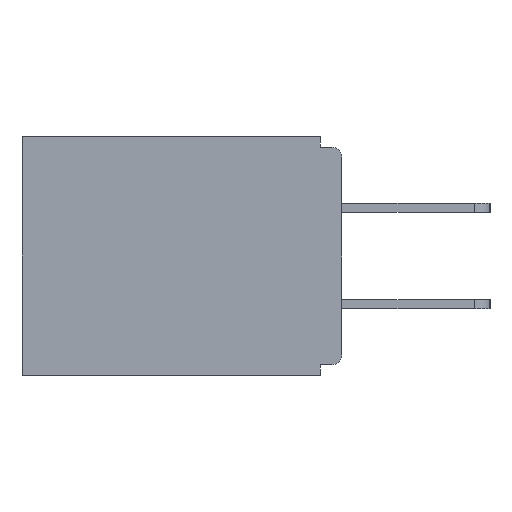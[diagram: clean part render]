
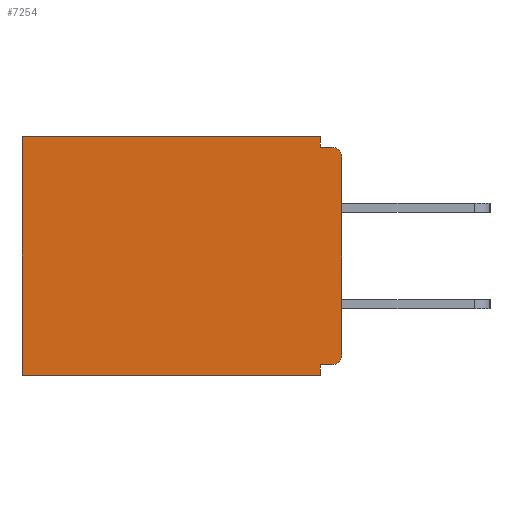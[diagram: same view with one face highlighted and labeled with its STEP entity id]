
A CAD part, left-side view. The second image highlights one B-rep face of the part: STEP entity #7254.
In plain terms, the highlighted planar face has unit normal (-1, 0, 0).
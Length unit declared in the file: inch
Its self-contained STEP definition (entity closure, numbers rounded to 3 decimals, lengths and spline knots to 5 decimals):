
#110 = VECTOR ( 'NONE', #3729, 39.37008 ) ;
#126 = VERTEX_POINT ( 'NONE', #10903 ) ;
#396 = DIRECTION ( 'NONE',  ( 1., 0., 0. ) ) ;
#443 = ORIENTED_EDGE ( 'NONE', *, *, #1362, .F. ) ;
#806 = CIRCLE ( 'NONE', #9338, 0.015 ) ;
#890 = VECTOR ( 'NONE', #6838, 39.37008 ) ;
#956 = VERTEX_POINT ( 'NONE', #1411 ) ;
#1042 = DIRECTION ( 'NONE',  ( 0., 1., 0. ) ) ;
#1362 = EDGE_CURVE ( 'NONE', #8880, #956, #7455, .T. ) ;
#1411 = CARTESIAN_POINT ( 'NONE',  ( 0.298, 0.015, -0.015 ) ) ;
#1448 = VERTEX_POINT ( 'NONE', #7820 ) ;
#1526 = AXIS2_PLACEMENT_3D ( 'NONE', #4943, #396, #4019 ) ;
#1796 = ORIENTED_EDGE ( 'NONE', *, *, #1849, .F. ) ;
#1849 = EDGE_CURVE ( 'NONE', #6363, #6569, #5545, .T. ) ;
#1912 = LINE ( 'NONE', #2779, #2485 ) ;
#1983 = CARTESIAN_POINT ( 'NONE',  ( 0.298, 0.015, -0.03 ) ) ;
#2081 = CARTESIAN_POINT ( 'NONE',  ( 0.298, 0., -0.343 ) ) ;
#2142 = CARTESIAN_POINT ( 'NONE',  ( 0.298, 0.031, -0.343 ) ) ;
#2427 = CARTESIAN_POINT ( 'NONE',  ( 0.298, 0.031, -0.328 ) ) ;
#2485 = VECTOR ( 'NONE', #1042, 39.37008 ) ;
#2779 = CARTESIAN_POINT ( 'NONE',  ( 0.298, 0., -0.328 ) ) ;
#3305 = ORIENTED_EDGE ( 'NONE', *, *, #5912, .F. ) ;
#3526 = DIRECTION ( 'NONE',  ( -1., 0., 0. ) ) ;
#3548 = EDGE_CURVE ( 'NONE', #1448, #8880, #4647, .T. ) ;
#3716 = AXIS2_PLACEMENT_3D ( 'NONE', #5342, #3526, #5758 ) ;
#3729 = DIRECTION ( 'NONE',  ( 0., 1., 0. ) ) ;
#3808 = CARTESIAN_POINT ( 'NONE',  ( 0.298, 0.015, -0.328 ) ) ;
#3820 = CIRCLE ( 'NONE', #3716, 0.015 ) ;
#3954 = CARTESIAN_POINT ( 'NONE',  ( 0.298, 0., -0.015 ) ) ;
#4019 = DIRECTION ( 'NONE',  ( 0., 0., -1. ) ) ;
#4382 = CARTESIAN_POINT ( 'NONE',  ( 0.298, 0., 0. ) ) ;
#4394 = VECTOR ( 'NONE', #4870, 39.37008 ) ;
#4421 = DIRECTION ( 'NONE',  ( 0., 0., -1. ) ) ;
#4441 = EDGE_CURVE ( 'NONE', #6363, #956, #806, .T. ) ;
#4455 = ORIENTED_EDGE ( 'NONE', *, *, #6949, .T. ) ;
#4647 = LINE ( 'NONE', #2142, #890 ) ;
#4870 = DIRECTION ( 'NONE',  ( 0., 0., -1. ) ) ;
#4943 = CARTESIAN_POINT ( 'NONE',  ( 0.298, 0., 0. ) ) ;
#4975 = VERTEX_POINT ( 'NONE', #8920 ) ;
#5342 = CARTESIAN_POINT ( 'NONE',  ( 0.298, 0.015, -0.313 ) ) ;
#5377 = EDGE_LOOP ( 'NONE', ( #6975, #443, #8109, #9449, #5841, #9059, #7332, #3305, #4455, #1796 ) ) ;
#5424 = CARTESIAN_POINT ( 'NONE',  ( 0.298, 0., -0.313 ) ) ;
#5545 = LINE ( 'NONE', #4382, #7303 ) ;
#5651 = CARTESIAN_POINT ( 'NONE',  ( 0.298, 0.031, -0.343 ) ) ;
#5711 = CARTESIAN_POINT ( 'NONE',  ( 0.298, 0.46, 0. ) ) ;
#5743 = CARTESIAN_POINT ( 'NONE',  ( 0.298, 0., -0.03 ) ) ;
#5758 = DIRECTION ( 'NONE',  ( 0., 0., -1. ) ) ;
#5841 = ORIENTED_EDGE ( 'NONE', *, *, #6872, .T. ) ;
#5912 = EDGE_CURVE ( 'NONE', #7705, #11423, #1912, .T. ) ;
#6060 = DIRECTION ( 'NONE',  ( 0., 1., 0. ) ) ;
#6061 = DIRECTION ( 'NONE',  ( 0., -1., 0. ) ) ;
#6254 = LINE ( 'NONE', #2081, #110 ) ;
#6363 = VERTEX_POINT ( 'NONE', #5743 ) ;
#6384 = EDGE_CURVE ( 'NONE', #126, #4975, #6254, .T. ) ;
#6502 = LINE ( 'NONE', #8766, #7724 ) ;
#6569 = VERTEX_POINT ( 'NONE', #5424 ) ;
#6838 = DIRECTION ( 'NONE',  ( 0., 0., -1. ) ) ;
#6872 = EDGE_CURVE ( 'NONE', #10521, #4975, #8308, .T. ) ;
#6949 = EDGE_CURVE ( 'NONE', #7705, #6569, #3820, .T. ) ;
#6975 = ORIENTED_EDGE ( 'NONE', *, *, #4441, .T. ) ;
#7254 = ADVANCED_FACE ( 'NONE', ( #9248 ), #9304, .F. ) ;
#7303 = VECTOR ( 'NONE', #4421, 39.37008 ) ;
#7315 = VECTOR ( 'NONE', #6061, 39.37008 ) ;
#7332 = ORIENTED_EDGE ( 'NONE', *, *, #9772, .F. ) ;
#7421 = VECTOR ( 'NONE', #8593, 39.37008 ) ;
#7455 = LINE ( 'NONE', #3954, #7315 ) ;
#7705 = VERTEX_POINT ( 'NONE', #3808 ) ;
#7724 = VECTOR ( 'NONE', #6060, 39.37008 ) ;
#7820 = CARTESIAN_POINT ( 'NONE',  ( 0.298, 0.031, 0. ) ) ;
#7972 = LINE ( 'NONE', #5651, #7421 ) ;
#8109 = ORIENTED_EDGE ( 'NONE', *, *, #3548, .F. ) ;
#8179 = DIRECTION ( 'NONE',  ( 0., 0., -1. ) ) ;
#8286 = EDGE_CURVE ( 'NONE', #1448, #10521, #6502, .T. ) ;
#8308 = LINE ( 'NONE', #5711, #4394 ) ;
#8593 = DIRECTION ( 'NONE',  ( 0., 0., -1. ) ) ;
#8766 = CARTESIAN_POINT ( 'NONE',  ( 0.298, 0., 0. ) ) ;
#8880 = VERTEX_POINT ( 'NONE', #9314 ) ;
#8920 = CARTESIAN_POINT ( 'NONE',  ( 0.298, 0.46, -0.343 ) ) ;
#9059 = ORIENTED_EDGE ( 'NONE', *, *, #6384, .F. ) ;
#9069 = DIRECTION ( 'NONE',  ( -1., 0., 0. ) ) ;
#9248 = FACE_OUTER_BOUND ( 'NONE', #5377, .T. ) ;
#9304 = PLANE ( 'NONE',  #1526 ) ;
#9314 = CARTESIAN_POINT ( 'NONE',  ( 0.298, 0.031, -0.015 ) ) ;
#9338 = AXIS2_PLACEMENT_3D ( 'NONE', #1983, #9069, #8179 ) ;
#9449 = ORIENTED_EDGE ( 'NONE', *, *, #8286, .T. ) ;
#9772 = EDGE_CURVE ( 'NONE', #11423, #126, #7972, .T. ) ;
#10381 = CARTESIAN_POINT ( 'NONE',  ( 0.298, 0.46, 0. ) ) ;
#10521 = VERTEX_POINT ( 'NONE', #10381 ) ;
#10903 = CARTESIAN_POINT ( 'NONE',  ( 0.298, 0.031, -0.343 ) ) ;
#11423 = VERTEX_POINT ( 'NONE', #2427 ) ;
